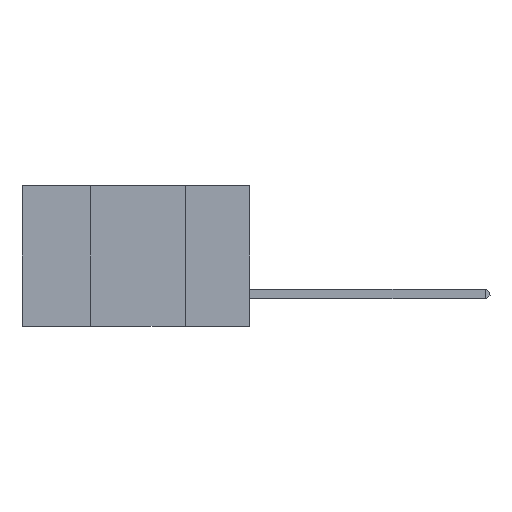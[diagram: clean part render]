
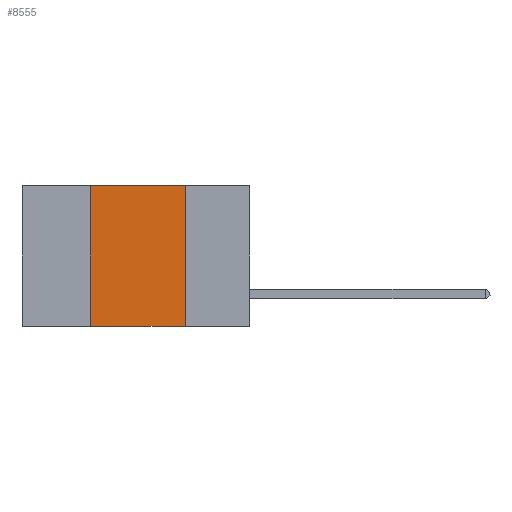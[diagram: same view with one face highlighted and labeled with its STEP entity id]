
A CAD part, left-side view. The second image highlights one B-rep face of the part: STEP entity #8555.
In plain terms, the highlighted planar face has unit normal (-1, 0, 0).
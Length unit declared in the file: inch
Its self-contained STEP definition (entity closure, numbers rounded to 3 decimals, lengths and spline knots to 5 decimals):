
#96 = PLANE ( 'NONE',  #10166 ) ;
#354 = ORIENTED_EDGE ( 'NONE', *, *, #8604, .F. ) ;
#1226 = DIRECTION ( 'NONE',  ( 0., 0., -1. ) ) ;
#1435 = VERTEX_POINT ( 'NONE', #7477 ) ;
#2624 = DIRECTION ( 'NONE',  ( 0., 0., -1. ) ) ;
#2672 = EDGE_CURVE ( 'NONE', #9016, #13609, #3567, .T. ) ;
#3502 = CARTESIAN_POINT ( 'NONE',  ( 0., 0.6, 0. ) ) ;
#3567 = LINE ( 'NONE', #9393, #3905 ) ;
#3650 = CARTESIAN_POINT ( 'NONE',  ( 0., 0.42, 0. ) ) ;
#3905 = VECTOR ( 'NONE', #7367, 39.37008 ) ;
#4414 = LINE ( 'NONE', #3650, #14142 ) ;
#5847 = CARTESIAN_POINT ( 'NONE',  ( 0., 0.6, 0. ) ) ;
#6223 = EDGE_CURVE ( 'NONE', #10286, #1435, #12733, .T. ) ;
#6970 = VECTOR ( 'NONE', #9382, 39.37008 ) ;
#7230 = ORIENTED_EDGE ( 'NONE', *, *, #2672, .T. ) ;
#7367 = DIRECTION ( 'NONE',  ( 0., -1., 0. ) ) ;
#7477 = CARTESIAN_POINT ( 'NONE',  ( 0., 0.17, 0. ) ) ;
#7647 = FACE_OUTER_BOUND ( 'NONE', #8017, .T. ) ;
#7882 = CARTESIAN_POINT ( 'NONE',  ( 0., 0.42, -0.37 ) ) ;
#7958 = DIRECTION ( 'NONE',  ( 1., 0., 0. ) ) ;
#8017 = EDGE_LOOP ( 'NONE', ( #354, #9647, #12520, #7230 ) ) ;
#8044 = CARTESIAN_POINT ( 'NONE',  ( 0., 0.42, 0. ) ) ;
#8358 = LINE ( 'NONE', #10209, #11330 ) ;
#8555 = ADVANCED_FACE ( 'NONE', ( #7647 ), #96, .F. ) ;
#8604 = EDGE_CURVE ( 'NONE', #1435, #13609, #8358, .T. ) ;
#8857 = CARTESIAN_POINT ( 'NONE',  ( 0., 0.17, -0.37 ) ) ;
#9016 = VERTEX_POINT ( 'NONE', #7882 ) ;
#9277 = DIRECTION ( 'NONE',  ( 0., 0., 1. ) ) ;
#9382 = DIRECTION ( 'NONE',  ( 0., -1., 0. ) ) ;
#9393 = CARTESIAN_POINT ( 'NONE',  ( 0., 0.6, -0.37 ) ) ;
#9647 = ORIENTED_EDGE ( 'NONE', *, *, #6223, .F. ) ;
#10166 = AXIS2_PLACEMENT_3D ( 'NONE', #3502, #7958, #1226 ) ;
#10209 = CARTESIAN_POINT ( 'NONE',  ( 0., 0.17, 0. ) ) ;
#10286 = VERTEX_POINT ( 'NONE', #8044 ) ;
#11330 = VECTOR ( 'NONE', #2624, 39.37008 ) ;
#12520 = ORIENTED_EDGE ( 'NONE', *, *, #13845, .F. ) ;
#12733 = LINE ( 'NONE', #5847, #6970 ) ;
#13609 = VERTEX_POINT ( 'NONE', #8857 ) ;
#13845 = EDGE_CURVE ( 'NONE', #9016, #10286, #4414, .T. ) ;
#14142 = VECTOR ( 'NONE', #9277, 39.37008 ) ;
